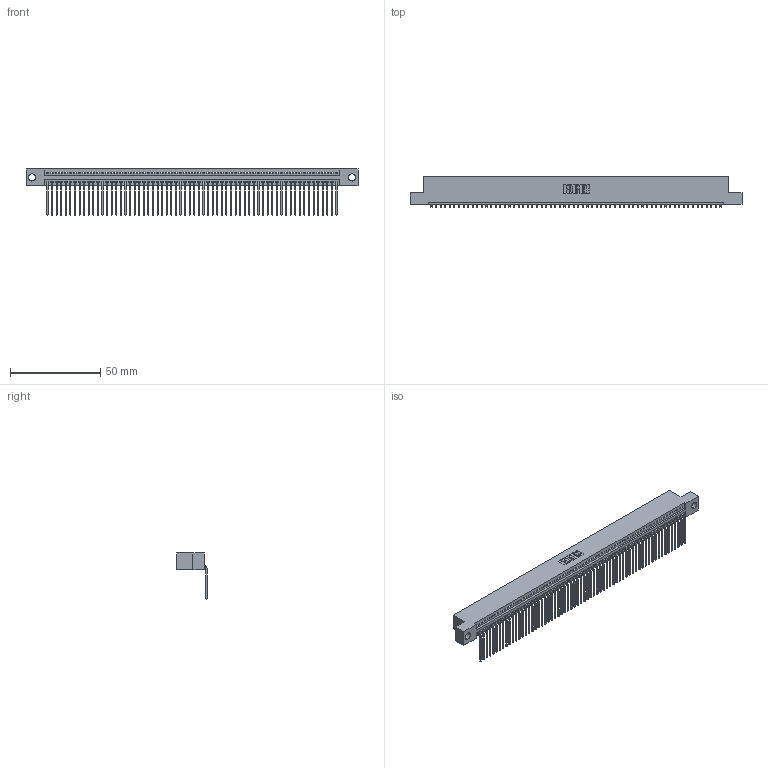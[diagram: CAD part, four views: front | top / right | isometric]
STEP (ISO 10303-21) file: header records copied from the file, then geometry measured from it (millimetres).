
FILE_DESCRIPTION (( 'STEP AP203' ), '1' );
FILE_NAME ('395-064-559-104.STEP', '2018-11-24T19:21:38', ( '' ), ( '' ), 'SwSTEP 2.0', 'SolidWorks 2016', '' );
FILE_SCHEMA (( 'CONFIG_CONTROL_DESIGN' ));
Length unit declared in the file: inch
Products named in the file (3): 345 Part_Flush Mounting Lugs - 0.156 Dia-TH; 345-292-001_558 559 Tail - 1; 395-064-559-104
Assembly tree (65 placements, depth 2):
  395-064-559-104
    345 Part_Flush Mounting Lugs - 0.156 Dia-TH
    345-292-001_558 559 Tail - 1  x64
Bounding box: 183.77 x 16.75 x 25.53 mm (x, y, z)
Volume: 17760.2 mm3; surface area: 24962.4 mm2
Topology: 65 solids, 65 shells, 3966 faces, 11989 edges, 7906 vertices
Faces by surface type: plane 2768, cylinder 1198
Entity records: 45293 total; most frequent: CARTESIAN_POINT 7852, ORIENTED_EDGE 7850, DIRECTION 6825, EDGE_CURVE 3925, VECTOR 3537, LINE 3537, VERTEX_POINT 2614, AXIS2_PLACEMENT_3D 1644
